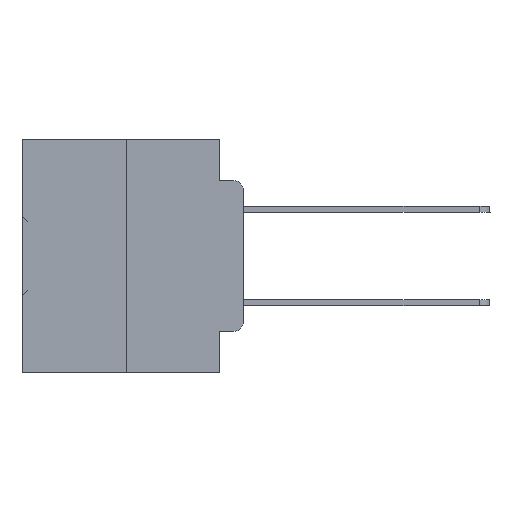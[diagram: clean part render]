
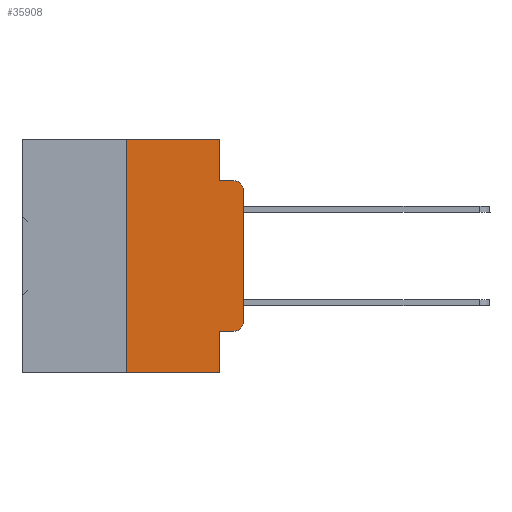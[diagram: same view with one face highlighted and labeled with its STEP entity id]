
A CAD part, left-side view. The second image highlights one B-rep face of the part: STEP entity #35908.
In plain terms, the highlighted planar face has unit normal (-1, 0, 0).
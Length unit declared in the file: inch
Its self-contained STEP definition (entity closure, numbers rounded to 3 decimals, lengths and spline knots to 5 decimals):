
#285 = VECTOR ( 'NONE', #12735, 39.37008 ) ;
#530 = AXIS2_PLACEMENT_3D ( 'NONE', #37327, #12253, #3365 ) ;
#773 = AXIS2_PLACEMENT_3D ( 'NONE', #35256, #4548, #4825 ) ;
#813 = EDGE_CURVE ( 'NONE', #28339, #10677, #17234, .T. ) ;
#1139 = CIRCLE ( 'NONE', #29374, 0.02 ) ;
#1308 = VERTEX_POINT ( 'NONE', #24551 ) ;
#1619 = CARTESIAN_POINT ( 'NONE',  ( 0., 0.051, 0. ) ) ;
#2311 = DIRECTION ( 'NONE',  ( 0., -1., 0. ) ) ;
#2758 = LINE ( 'NONE', #32095, #36149 ) ;
#3365 = DIRECTION ( 'NONE',  ( 0., 0., -1. ) ) ;
#4548 = DIRECTION ( 'NONE',  ( -1., 0., 0. ) ) ;
#4825 = DIRECTION ( 'NONE',  ( 0., 0., -1. ) ) ;
#4853 = DIRECTION ( 'NONE',  ( 0., 0., -1. ) ) ;
#5453 = VERTEX_POINT ( 'NONE', #24301 ) ;
#5721 = VERTEX_POINT ( 'NONE', #23124 ) ;
#6248 = ORIENTED_EDGE ( 'NONE', *, *, #20564, .F. ) ;
#7058 = VECTOR ( 'NONE', #2311, 39.37008 ) ;
#7416 = LINE ( 'NONE', #1619, #21937 ) ;
#7566 = ORIENTED_EDGE ( 'NONE', *, *, #813, .F. ) ;
#7907 = CARTESIAN_POINT ( 'NONE',  ( 0., 0., -0.1085 ) ) ;
#8869 = ORIENTED_EDGE ( 'NONE', *, *, #10714, .T. ) ;
#9220 = VECTOR ( 'NONE', #26197, 39.37008 ) ;
#10239 = VERTEX_POINT ( 'NONE', #7907 ) ;
#10677 = VERTEX_POINT ( 'NONE', #31997 ) ;
#10714 = EDGE_CURVE ( 'NONE', #1308, #5721, #1139, .T. ) ;
#11032 = ORIENTED_EDGE ( 'NONE', *, *, #20659, .F. ) ;
#11147 = DIRECTION ( 'NONE',  ( -1., 0., 0. ) ) ;
#12188 = EDGE_CURVE ( 'NONE', #38883, #1308, #2758, .T. ) ;
#12253 = DIRECTION ( 'NONE',  ( 1., 0., 0. ) ) ;
#12430 = CARTESIAN_POINT ( 'NONE',  ( 0., 0.051, 0. ) ) ;
#12505 = PLANE ( 'NONE',  #530 ) ;
#12735 = DIRECTION ( 'NONE',  ( 0., 0., 1. ) ) ;
#13127 = EDGE_CURVE ( 'NONE', #38883, #32671, #7416, .T. ) ;
#13703 = CARTESIAN_POINT ( 'NONE',  ( 0., 0.051, -0.0885 ) ) ;
#17182 = CARTESIAN_POINT ( 'NONE',  ( 0., 0.473, -0.5 ) ) ;
#17234 = LINE ( 'NONE', #24877, #285 ) ;
#17600 = DIRECTION ( 'NONE',  ( 0., -1., 0. ) ) ;
#17606 = CARTESIAN_POINT ( 'NONE',  ( 0., 0.02, -0.0885 ) ) ;
#18782 = ORIENTED_EDGE ( 'NONE', *, *, #12188, .T. ) ;
#18863 = EDGE_CURVE ( 'NONE', #10239, #27148, #25709, .T. ) ;
#19225 = VECTOR ( 'NONE', #25481, 39.37008 ) ;
#20564 = EDGE_CURVE ( 'NONE', #10677, #24714, #29506, .T. ) ;
#20659 = EDGE_CURVE ( 'NONE', #24714, #5453, #37015, .T. ) ;
#21578 = EDGE_CURVE ( 'NONE', #5453, #27148, #35163, .T. ) ;
#21937 = VECTOR ( 'NONE', #4853, 39.37008 ) ;
#22332 = CARTESIAN_POINT ( 'NONE',  ( 0., 0.473, 0. ) ) ;
#22900 = CARTESIAN_POINT ( 'NONE',  ( 0., 0., 0. ) ) ;
#22933 = LINE ( 'NONE', #17182, #28292 ) ;
#23124 = CARTESIAN_POINT ( 'NONE',  ( 0., 0., -0.3915 ) ) ;
#23417 = CARTESIAN_POINT ( 'NONE',  ( 0., 0.051, -0.5 ) ) ;
#23941 = VECTOR ( 'NONE', #31967, 39.37008 ) ;
#24301 = CARTESIAN_POINT ( 'NONE',  ( 0., 0.051, -0.0885 ) ) ;
#24551 = CARTESIAN_POINT ( 'NONE',  ( 0., 0.02, -0.4115 ) ) ;
#24657 = FACE_OUTER_BOUND ( 'NONE', #34388, .T. ) ;
#24714 = VERTEX_POINT ( 'NONE', #12430 ) ;
#24877 = CARTESIAN_POINT ( 'NONE',  ( 0., 0.25, 0. ) ) ;
#25052 = EDGE_CURVE ( 'NONE', #28339, #32671, #22933, .T. ) ;
#25481 = DIRECTION ( 'NONE',  ( 0., -1., 0. ) ) ;
#25709 = CIRCLE ( 'NONE', #773, 0.02 ) ;
#25736 = DIRECTION ( 'NONE',  ( 0., -1., 0. ) ) ;
#26197 = DIRECTION ( 'NONE',  ( 0., 0., 1. ) ) ;
#26631 = CARTESIAN_POINT ( 'NONE',  ( 0., 0.02, -0.3915 ) ) ;
#26696 = LINE ( 'NONE', #22900, #9220 ) ;
#27148 = VERTEX_POINT ( 'NONE', #17606 ) ;
#28292 = VECTOR ( 'NONE', #17600, 39.37008 ) ;
#28339 = VERTEX_POINT ( 'NONE', #33535 ) ;
#28553 = ORIENTED_EDGE ( 'NONE', *, *, #21578, .F. ) ;
#29374 = AXIS2_PLACEMENT_3D ( 'NONE', #26631, #11147, #38921 ) ;
#29506 = LINE ( 'NONE', #22332, #19225 ) ;
#29938 = ORIENTED_EDGE ( 'NONE', *, *, #25052, .T. ) ;
#31315 = CARTESIAN_POINT ( 'NONE',  ( 0., 0.051, -0.4115 ) ) ;
#31829 = ORIENTED_EDGE ( 'NONE', *, *, #13127, .F. ) ;
#31836 = CARTESIAN_POINT ( 'NONE',  ( 0., 0.051, 0. ) ) ;
#31967 = DIRECTION ( 'NONE',  ( 0., 0., -1. ) ) ;
#31997 = CARTESIAN_POINT ( 'NONE',  ( 0., 0.25, 0. ) ) ;
#32095 = CARTESIAN_POINT ( 'NONE',  ( 0., 0.051, -0.4115 ) ) ;
#32671 = VERTEX_POINT ( 'NONE', #23417 ) ;
#33535 = CARTESIAN_POINT ( 'NONE',  ( 0., 0.25, -0.5 ) ) ;
#34388 = EDGE_LOOP ( 'NONE', ( #39154, #39628, #28553, #11032, #6248, #7566, #29938, #31829, #18782, #8869 ) ) ;
#35163 = LINE ( 'NONE', #13703, #7058 ) ;
#35256 = CARTESIAN_POINT ( 'NONE',  ( 0., 0.02, -0.1085 ) ) ;
#35908 = ADVANCED_FACE ( 'NONE', ( #24657 ), #12505, .F. ) ;
#36149 = VECTOR ( 'NONE', #25736, 39.37008 ) ;
#37015 = LINE ( 'NONE', #31836, #23941 ) ;
#37327 = CARTESIAN_POINT ( 'NONE',  ( 0., 0.473, 0. ) ) ;
#38883 = VERTEX_POINT ( 'NONE', #31315 ) ;
#38921 = DIRECTION ( 'NONE',  ( 0., 0., -1. ) ) ;
#39026 = EDGE_CURVE ( 'NONE', #5721, #10239, #26696, .T. ) ;
#39154 = ORIENTED_EDGE ( 'NONE', *, *, #39026, .T. ) ;
#39628 = ORIENTED_EDGE ( 'NONE', *, *, #18863, .T. ) ;
